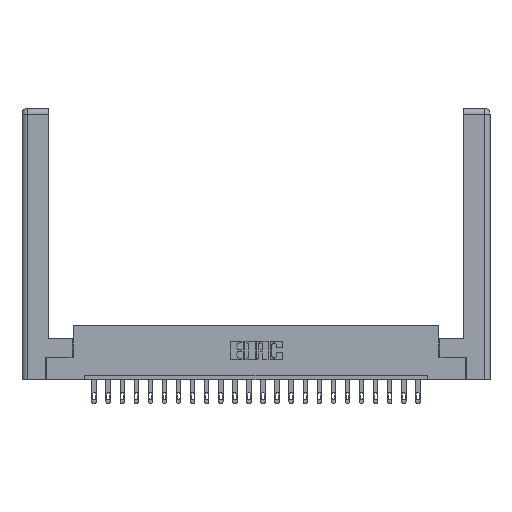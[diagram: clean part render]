
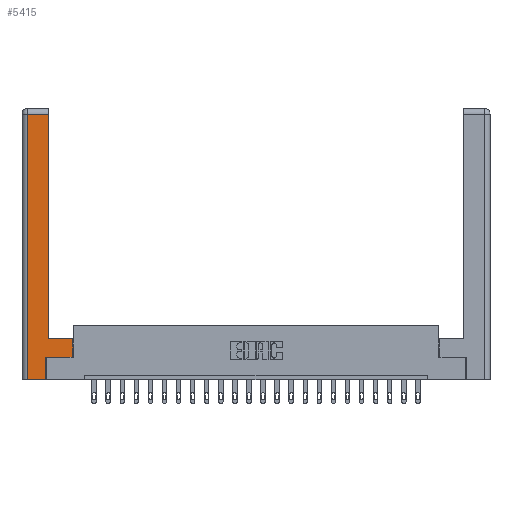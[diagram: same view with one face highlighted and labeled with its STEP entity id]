
A CAD part, top view. The second image highlights one B-rep face of the part: STEP entity #5415.
In plain terms, the highlighted planar face has unit normal (0, 0, 1).
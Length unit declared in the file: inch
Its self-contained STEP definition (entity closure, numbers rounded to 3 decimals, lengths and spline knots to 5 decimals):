
#80 = CARTESIAN_POINT ( 'NONE',  ( 0.265, 0., 0. ) ) ;
#373 = LINE ( 'NONE', #12306, #11079 ) ;
#577 = VERTEX_POINT ( 'NONE', #22291 ) ;
#901 = VERTEX_POINT ( 'NONE', #13815 ) ;
#1802 = DIRECTION ( 'NONE',  ( 0., -1., 0. ) ) ;
#2374 = EDGE_CURVE ( 'NONE', #7859, #577, #19675, .T. ) ;
#2660 = FACE_OUTER_BOUND ( 'NONE', #6605, .T. ) ;
#3465 = EDGE_CURVE ( 'NONE', #9953, #14305, #5324, .T. ) ;
#4675 = VERTEX_POINT ( 'NONE', #20977 ) ;
#5306 = DIRECTION ( 'NONE',  ( 1., 0., 0. ) ) ;
#5324 = LINE ( 'NONE', #14371, #21003 ) ;
#5338 = CARTESIAN_POINT ( 'NONE',  ( 0., 0., 0. ) ) ;
#5346 = CARTESIAN_POINT ( 'NONE',  ( 0.565, 0.45, 0. ) ) ;
#5415 = ADVANCED_FACE ( 'NONE', ( #2660 ), #13943, .F. ) ;
#5666 = VECTOR ( 'NONE', #15977, 39.37008 ) ;
#5947 = ORIENTED_EDGE ( 'NONE', *, *, #16605, .T. ) ;
#6253 = EDGE_CURVE ( 'NONE', #14305, #7699, #14959, .T. ) ;
#6605 = EDGE_LOOP ( 'NONE', ( #11341, #22310, #10988, #17145, #5947, #21135, #9077, #6832 ) ) ;
#6764 = LINE ( 'NONE', #7625, #20222 ) ;
#6832 = ORIENTED_EDGE ( 'NONE', *, *, #2374, .T. ) ;
#7625 = CARTESIAN_POINT ( 'NONE',  ( 0.565, 0.45, 0. ) ) ;
#7699 = VERTEX_POINT ( 'NONE', #13257 ) ;
#7853 = DIRECTION ( 'NONE',  ( 0., 1., 0. ) ) ;
#7859 = VERTEX_POINT ( 'NONE', #5346 ) ;
#8812 = DIRECTION ( 'NONE',  ( -1., 0., 0. ) ) ;
#9077 = ORIENTED_EDGE ( 'NONE', *, *, #16162, .T. ) ;
#9953 = VERTEX_POINT ( 'NONE', #14833 ) ;
#9962 = CARTESIAN_POINT ( 'NONE',  ( 0.265, 0., 0. ) ) ;
#10182 = DIRECTION ( 'NONE',  ( 1., 0., 0. ) ) ;
#10988 = ORIENTED_EDGE ( 'NONE', *, *, #6253, .T. ) ;
#11079 = VECTOR ( 'NONE', #5306, 39.37008 ) ;
#11341 = ORIENTED_EDGE ( 'NONE', *, *, #11942, .T. ) ;
#11785 = CARTESIAN_POINT ( 'NONE',  ( 0.0615, 2.94, 0. ) ) ;
#11927 = EDGE_CURVE ( 'NONE', #4675, #901, #373, .T. ) ;
#11942 = EDGE_CURVE ( 'NONE', #577, #9953, #17099, .T. ) ;
#12306 = CARTESIAN_POINT ( 'NONE',  ( 0.565, 0.245, 0. ) ) ;
#12755 = CARTESIAN_POINT ( 'NONE',  ( 0.265, 0.245, 0. ) ) ;
#13038 = LINE ( 'NONE', #12755, #19372 ) ;
#13257 = CARTESIAN_POINT ( 'NONE',  ( 0.0615, 0., 0. ) ) ;
#13621 = LINE ( 'NONE', #9962, #14196 ) ;
#13815 = CARTESIAN_POINT ( 'NONE',  ( 0.565, 0.245, 0. ) ) ;
#13943 = PLANE ( 'NONE',  #18249 ) ;
#14075 = CARTESIAN_POINT ( 'NONE',  ( 0.295, 0.45, 0. ) ) ;
#14196 = VECTOR ( 'NONE', #10182, 39.37008 ) ;
#14305 = VERTEX_POINT ( 'NONE', #11785 ) ;
#14371 = CARTESIAN_POINT ( 'NONE',  ( 0.0615, 2.94, 0. ) ) ;
#14505 = DIRECTION ( 'NONE',  ( 0., 1., 0. ) ) ;
#14654 = CARTESIAN_POINT ( 'NONE',  ( 0.295, 3., 0. ) ) ;
#14833 = CARTESIAN_POINT ( 'NONE',  ( 0.295, 2.94, 0. ) ) ;
#14959 = LINE ( 'NONE', #15822, #14979 ) ;
#14979 = VECTOR ( 'NONE', #1802, 39.37008 ) ;
#15774 = EDGE_CURVE ( 'NONE', #7699, #21896, #13621, .T. ) ;
#15822 = CARTESIAN_POINT ( 'NONE',  ( 0.0615, 0., 0. ) ) ;
#15977 = DIRECTION ( 'NONE',  ( -1., 0., 0. ) ) ;
#16016 = VECTOR ( 'NONE', #17962, 39.37008 ) ;
#16162 = EDGE_CURVE ( 'NONE', #901, #7859, #6764, .T. ) ;
#16605 = EDGE_CURVE ( 'NONE', #21896, #4675, #13038, .T. ) ;
#17099 = LINE ( 'NONE', #14654, #16016 ) ;
#17145 = ORIENTED_EDGE ( 'NONE', *, *, #15774, .T. ) ;
#17544 = DIRECTION ( 'NONE',  ( 0., 0., -1. ) ) ;
#17904 = DIRECTION ( 'NONE',  ( -1., 0., 0. ) ) ;
#17962 = DIRECTION ( 'NONE',  ( 0., 1., 0. ) ) ;
#18249 = AXIS2_PLACEMENT_3D ( 'NONE', #5338, #17544, #8812 ) ;
#19372 = VECTOR ( 'NONE', #14505, 39.37008 ) ;
#19675 = LINE ( 'NONE', #14075, #5666 ) ;
#20222 = VECTOR ( 'NONE', #7853, 39.37008 ) ;
#20977 = CARTESIAN_POINT ( 'NONE',  ( 0.265, 0.245, 0. ) ) ;
#21003 = VECTOR ( 'NONE', #17904, 39.37008 ) ;
#21135 = ORIENTED_EDGE ( 'NONE', *, *, #11927, .T. ) ;
#21896 = VERTEX_POINT ( 'NONE', #80 ) ;
#22291 = CARTESIAN_POINT ( 'NONE',  ( 0.295, 0.45, 0. ) ) ;
#22310 = ORIENTED_EDGE ( 'NONE', *, *, #3465, .T. ) ;
